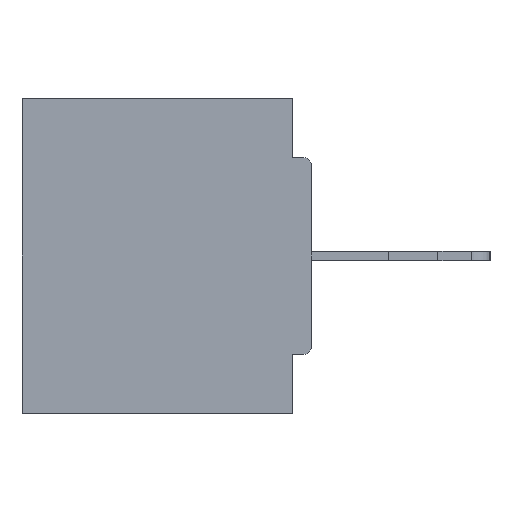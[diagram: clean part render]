
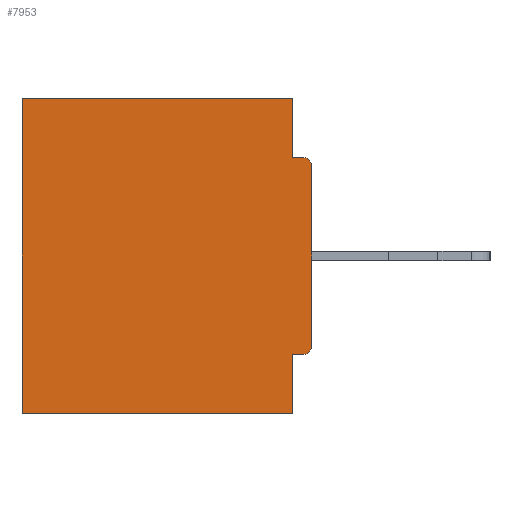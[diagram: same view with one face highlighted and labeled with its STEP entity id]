
A CAD part, left-side view. The second image highlights one B-rep face of the part: STEP entity #7953.
In plain terms, the highlighted planar face has unit normal (-1, 0, 0).
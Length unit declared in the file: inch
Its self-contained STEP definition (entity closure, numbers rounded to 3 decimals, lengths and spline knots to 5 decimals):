
#146 = ORIENTED_EDGE ( 'NONE', *, *, #17272, .T. ) ;
#198 = CARTESIAN_POINT ( 'NONE',  ( 0.298, 0.031, -0.5 ) ) ;
#494 = LINE ( 'NONE', #30055, #6361 ) ;
#571 = CARTESIAN_POINT ( 'NONE',  ( 0.298, 0.031, -0.4065 ) ) ;
#582 = VERTEX_POINT ( 'NONE', #571 ) ;
#1016 = ORIENTED_EDGE ( 'NONE', *, *, #20102, .T. ) ;
#1077 = ORIENTED_EDGE ( 'NONE', *, *, #27016, .F. ) ;
#1323 = LINE ( 'NONE', #20175, #13561 ) ;
#1413 = DIRECTION ( 'NONE',  ( 0., 1., 0. ) ) ;
#1683 = LINE ( 'NONE', #29312, #13891 ) ;
#1996 = LINE ( 'NONE', #8257, #14189 ) ;
#2158 = PLANE ( 'NONE',  #30017 ) ;
#2359 = VERTEX_POINT ( 'NONE', #25117 ) ;
#2876 = DIRECTION ( 'NONE',  ( 0., 1., 0. ) ) ;
#4213 = CARTESIAN_POINT ( 'NONE',  ( 0.298, 0.031, -0.5 ) ) ;
#4970 = CARTESIAN_POINT ( 'NONE',  ( 0.298, 0., 0. ) ) ;
#5557 = CARTESIAN_POINT ( 'NONE',  ( 0.298, 0., -0.3915 ) ) ;
#5860 = EDGE_CURVE ( 'NONE', #27135, #9004, #494, .T. ) ;
#6361 = VECTOR ( 'NONE', #12684, 39.37008 ) ;
#6515 = ORIENTED_EDGE ( 'NONE', *, *, #27184, .F. ) ;
#6582 = EDGE_CURVE ( 'NONE', #15803, #26324, #13135, .T. ) ;
#6691 = DIRECTION ( 'NONE',  ( 0., 0., -1. ) ) ;
#6948 = ORIENTED_EDGE ( 'NONE', *, *, #15178, .F. ) ;
#7806 = EDGE_CURVE ( 'NONE', #15803, #21271, #27402, .T. ) ;
#7953 = ADVANCED_FACE ( 'NONE', ( #29106 ), #2158, .F. ) ;
#8257 = CARTESIAN_POINT ( 'NONE',  ( 0.298, 0., -0.0935 ) ) ;
#9004 = VERTEX_POINT ( 'NONE', #29058 ) ;
#10776 = VERTEX_POINT ( 'NONE', #198 ) ;
#11670 = DIRECTION ( 'NONE',  ( -1., 0., 0. ) ) ;
#12349 = VERTEX_POINT ( 'NONE', #19907 ) ;
#12619 = VECTOR ( 'NONE', #2876, 39.37008 ) ;
#12684 = DIRECTION ( 'NONE',  ( 0., 0., -1. ) ) ;
#13135 = LINE ( 'NONE', #20746, #18510 ) ;
#13237 = VERTEX_POINT ( 'NONE', #14367 ) ;
#13328 = ORIENTED_EDGE ( 'NONE', *, *, #29256, .F. ) ;
#13561 = VECTOR ( 'NONE', #22433, 39.37008 ) ;
#13891 = VECTOR ( 'NONE', #1413, 39.37008 ) ;
#14156 = DIRECTION ( 'NONE',  ( -1., 0., 0. ) ) ;
#14189 = VECTOR ( 'NONE', #28851, 39.37008 ) ;
#14367 = CARTESIAN_POINT ( 'NONE',  ( 0.298, 0.015, -0.4065 ) ) ;
#14654 = CIRCLE ( 'NONE', #22240, 0.015 ) ;
#15012 = AXIS2_PLACEMENT_3D ( 'NONE', #24018, #14156, #22947 ) ;
#15123 = ORIENTED_EDGE ( 'NONE', *, *, #7806, .T. ) ;
#15178 = EDGE_CURVE ( 'NONE', #13237, #582, #18735, .T. ) ;
#15513 = DIRECTION ( 'NONE',  ( 1., 0., 0. ) ) ;
#15711 = DIRECTION ( 'NONE',  ( 0., 0., -1. ) ) ;
#15803 = VERTEX_POINT ( 'NONE', #19611 ) ;
#17272 = EDGE_CURVE ( 'NONE', #13237, #26324, #14654, .T. ) ;
#18510 = VECTOR ( 'NONE', #15711, 39.37008 ) ;
#18735 = LINE ( 'NONE', #26187, #12619 ) ;
#19611 = CARTESIAN_POINT ( 'NONE',  ( 0.298, 0., -0.1085 ) ) ;
#19907 = CARTESIAN_POINT ( 'NONE',  ( 0.298, 0.46, -0.5 ) ) ;
#20102 = EDGE_CURVE ( 'NONE', #2359, #12349, #29263, .T. ) ;
#20175 = CARTESIAN_POINT ( 'NONE',  ( 0.298, 0., -0.5 ) ) ;
#20733 = VECTOR ( 'NONE', #6691, 39.37008 ) ;
#20746 = CARTESIAN_POINT ( 'NONE',  ( 0.298, 0., 0. ) ) ;
#21271 = VERTEX_POINT ( 'NONE', #28624 ) ;
#21418 = LINE ( 'NONE', #4213, #20733 ) ;
#22240 = AXIS2_PLACEMENT_3D ( 'NONE', #25334, #11670, #27525 ) ;
#22433 = DIRECTION ( 'NONE',  ( 0., 1., 0. ) ) ;
#22681 = ORIENTED_EDGE ( 'NONE', *, *, #6582, .F. ) ;
#22711 = VECTOR ( 'NONE', #23650, 39.37008 ) ;
#22947 = DIRECTION ( 'NONE',  ( 0., 0., -1. ) ) ;
#23650 = DIRECTION ( 'NONE',  ( 0., 0., -1. ) ) ;
#24018 = CARTESIAN_POINT ( 'NONE',  ( 0.298, 0.015, -0.1085 ) ) ;
#25117 = CARTESIAN_POINT ( 'NONE',  ( 0.298, 0.46, 0. ) ) ;
#25312 = DIRECTION ( 'NONE',  ( 0., 0., -1. ) ) ;
#25334 = CARTESIAN_POINT ( 'NONE',  ( 0.298, 0.015, -0.3915 ) ) ;
#26019 = EDGE_LOOP ( 'NONE', ( #15123, #13328, #26925, #30217, #1016, #1077, #6515, #6948, #146, #22681 ) ) ;
#26187 = CARTESIAN_POINT ( 'NONE',  ( 0.298, 0., -0.4065 ) ) ;
#26324 = VERTEX_POINT ( 'NONE', #5557 ) ;
#26925 = ORIENTED_EDGE ( 'NONE', *, *, #5860, .F. ) ;
#27016 = EDGE_CURVE ( 'NONE', #10776, #12349, #1323, .T. ) ;
#27135 = VERTEX_POINT ( 'NONE', #27248 ) ;
#27184 = EDGE_CURVE ( 'NONE', #582, #10776, #21418, .T. ) ;
#27248 = CARTESIAN_POINT ( 'NONE',  ( 0.298, 0.031, 0. ) ) ;
#27402 = CIRCLE ( 'NONE', #15012, 0.015 ) ;
#27525 = DIRECTION ( 'NONE',  ( 0., 0., -1. ) ) ;
#28012 = CARTESIAN_POINT ( 'NONE',  ( 0.298, 0.46, 0. ) ) ;
#28263 = EDGE_CURVE ( 'NONE', #27135, #2359, #1683, .T. ) ;
#28624 = CARTESIAN_POINT ( 'NONE',  ( 0.298, 0.015, -0.0935 ) ) ;
#28851 = DIRECTION ( 'NONE',  ( 0., -1., 0. ) ) ;
#29058 = CARTESIAN_POINT ( 'NONE',  ( 0.298, 0.031, -0.0935 ) ) ;
#29106 = FACE_OUTER_BOUND ( 'NONE', #26019, .T. ) ;
#29256 = EDGE_CURVE ( 'NONE', #9004, #21271, #1996, .T. ) ;
#29263 = LINE ( 'NONE', #28012, #22711 ) ;
#29312 = CARTESIAN_POINT ( 'NONE',  ( 0.298, 0., 0. ) ) ;
#30017 = AXIS2_PLACEMENT_3D ( 'NONE', #4970, #15513, #25312 ) ;
#30055 = CARTESIAN_POINT ( 'NONE',  ( 0.298, 0.031, -0.5 ) ) ;
#30217 = ORIENTED_EDGE ( 'NONE', *, *, #28263, .T. ) ;
